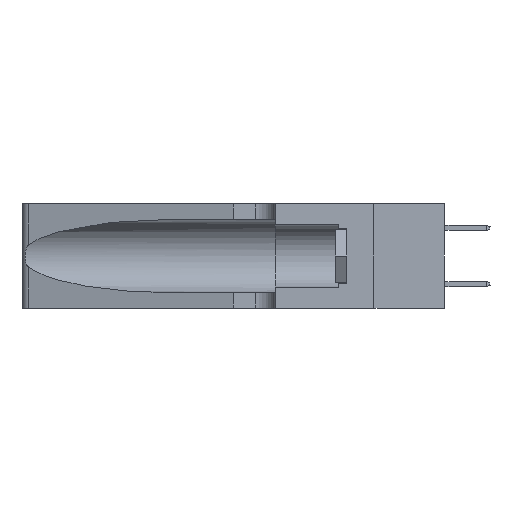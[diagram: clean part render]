
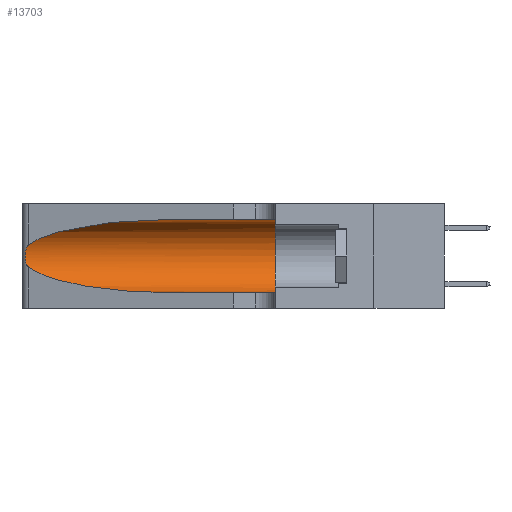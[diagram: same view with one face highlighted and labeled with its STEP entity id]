
A CAD part, left-side view. The second image highlights one B-rep face of the part: STEP entity #13703.
In plain terms, the highlighted cylindrical face has radius 3.308 mm (diameter 6.617 mm), a partial arc.
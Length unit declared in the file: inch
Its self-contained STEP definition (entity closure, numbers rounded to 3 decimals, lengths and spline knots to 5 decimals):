
#345 = ORIENTED_EDGE ( 'NONE', *, *, #11980, .T. ) ;
#488 = VECTOR ( 'NONE', #24105, 39.37008 ) ;
#1249 = CARTESIAN_POINT ( 'NONE',  ( 0.25856, 1.23593, 0.16098 ) ) ;
#1581 = CARTESIAN_POINT ( 'NONE',  ( 0.25639, 1.23184, 0.21858 ) ) ;
#1727 = DIRECTION ( 'NONE',  ( 0., -1., 0. ) ) ;
#2089 = VERTEX_POINT ( 'NONE', #17372 ) ;
#2614 = AXIS2_PLACEMENT_3D ( 'NONE', #23017, #25202, #8219 ) ;
#2866 = CIRCLE ( 'NONE', #2614, 0.13025 ) ;
#4039 = CARTESIAN_POINT ( 'NONE',  ( 0.25789, 1.23486, 0.15765 ) ) ;
#4110 = EDGE_CURVE ( 'NONE', #21217, #9822, #2866, .T. ) ;
#4448 = CARTESIAN_POINT ( 'NONE',  ( 0.2373, 1.15595, 0.08982 ) ) ;
#4817 = CARTESIAN_POINT ( 'NONE',  ( 0.1305, 1.61858, 0.31525 ) ) ;
#6297 = CARTESIAN_POINT ( 'NONE',  ( 0.1305, 0.72297, 0.31525 ) ) ;
#7261 = ORIENTED_EDGE ( 'NONE', *, *, #7979, .F. ) ;
#7979 = EDGE_CURVE ( 'NONE', #8093, #21217, #15474, .T. ) ;
#8093 = VERTEX_POINT ( 'NONE', #6297 ) ;
#8219 = DIRECTION ( 'NONE',  ( 0., 0., 1. ) ) ;
#9145 = CARTESIAN_POINT ( 'NONE',  ( 0.26075, 1.23896, 0.178 ) ) ;
#9822 = VERTEX_POINT ( 'NONE', #28395 ) ;
#11286 = EDGE_CURVE ( 'NONE', #16713, #2089, #21989, .T. ) ;
#11312 = CARTESIAN_POINT ( 'NONE',  ( 0.25555, 1.22994, 0.2215 ) ) ;
#11980 = EDGE_CURVE ( 'NONE', #2089, #9822, #21473, .T. ) ;
#12191 = ORIENTED_EDGE ( 'NONE', *, *, #4110, .F. ) ;
#13606 = DIRECTION ( 'NONE',  ( 0., 0., -1. ) ) ;
#13671 = CARTESIAN_POINT ( 'NONE',  ( 0.25487, 1.22718, 0.22369 ) ) ;
#13703 = ADVANCED_FACE ( 'NONE', ( #27116 ), #22450, .F. ) ;
#13953 = ORIENTED_EDGE ( 'NONE', *, *, #21224, .T. ) ;
#14347 = CARTESIAN_POINT ( 'NONE',  ( 0.25487, 1.22718, 0.14631 ) ) ;
#14461 = CARTESIAN_POINT ( 'NONE',  ( 0.25639, 1.23186, 0.15144 ) ) ;
#15474 = LINE ( 'NONE', #4817, #21306 ) ;
#16266 =( BOUNDED_CURVE ( )  B_SPLINE_CURVE ( 3, ( #28677, #31239, #18958, #13671 ),
 .UNSPECIFIED., .F., .T. ) 
 B_SPLINE_CURVE_WITH_KNOTS ( ( 4, 4 ),
 ( 1.5708, 2.84003 ),
 .UNSPECIFIED. ) 
 CURVE ( )  GEOMETRIC_REPRESENTATION_ITEM ( )  RATIONAL_B_SPLINE_CURVE ( ( 1., 0.87, 0.87, 1. ) ) 
 REPRESENTATION_ITEM ( '' )  );
#16453 = CARTESIAN_POINT ( 'NONE',  ( 0.25487, 1.22718, 0.14631 ) ) ;
#16506 = CARTESIAN_POINT ( 'NONE',  ( 0.1305, 0.35, 0.31525 ) ) ;
#16713 = VERTEX_POINT ( 'NONE', #16453 ) ;
#17372 = CARTESIAN_POINT ( 'NONE',  ( 0.1305, 0.72297, 0.05475 ) ) ;
#18273 = ORIENTED_EDGE ( 'NONE', *, *, #24358, .T. ) ;
#18329 = CARTESIAN_POINT ( 'NONE',  ( 0.1305, 1.61858, 0.05475 ) ) ;
#18750 = CARTESIAN_POINT ( 'NONE',  ( 0.25854, 1.2359, 0.20912 ) ) ;
#18866 = CARTESIAN_POINT ( 'NONE',  ( 0.26075, 1.23896, 0.19203 ) ) ;
#18958 = CARTESIAN_POINT ( 'NONE',  ( 0.2373, 1.15595, 0.28018 ) ) ;
#19444 = B_SPLINE_CURVE_WITH_KNOTS ( 'NONE', 3,
 ( #21134, #11312, #1581, #23953, #18750, #21249, #18866, #9145, #26433, #1249, #4039, #14461, #29241, #14347 ),
 .UNSPECIFIED., .F., .F.,
 ( 4, 2, 2, 2, 2, 2, 4 ),
 ( 0., 0.00027, 0.00053, 0.00107, 0.0016, 0.00187, 0.00214 ),
 .UNSPECIFIED. ) ;
#21134 = CARTESIAN_POINT ( 'NONE',  ( 0.25487, 1.22718, 0.22369 ) ) ;
#21217 = VERTEX_POINT ( 'NONE', #16506 ) ;
#21224 = EDGE_CURVE ( 'NONE', #8093, #24990, #16266, .T. ) ;
#21249 = CARTESIAN_POINT ( 'NONE',  ( 0.26018, 1.23835, 0.19895 ) ) ;
#21306 = VECTOR ( 'NONE', #30594, 39.37008 ) ;
#21473 = LINE ( 'NONE', #18329, #488 ) ;
#21702 = CARTESIAN_POINT ( 'NONE',  ( 0.25487, 1.22718, 0.22369 ) ) ;
#21989 =( BOUNDED_CURVE ( )  B_SPLINE_CURVE ( 3, ( #26277, #4448, #26392, #24242 ),
 .UNSPECIFIED., .F., .F. ) 
 B_SPLINE_CURVE_WITH_KNOTS ( ( 4, 4 ),
 ( 3.44316, 4.71239 ),
 .UNSPECIFIED. ) 
 CURVE ( )  GEOMETRIC_REPRESENTATION_ITEM ( )  RATIONAL_B_SPLINE_CURVE ( ( 1., 0.87, 0.87, 1. ) ) 
 REPRESENTATION_ITEM ( '' )  );
#22450 = CYLINDRICAL_SURFACE ( 'NONE', #23527, 0.13025 ) ;
#23017 = CARTESIAN_POINT ( 'NONE',  ( 0.1305, 0.35, 0.185 ) ) ;
#23527 = AXIS2_PLACEMENT_3D ( 'NONE', #28734, #1727, #13606 ) ;
#23953 = CARTESIAN_POINT ( 'NONE',  ( 0.25787, 1.23484, 0.2124 ) ) ;
#24105 = DIRECTION ( 'NONE',  ( 0., -1., 0. ) ) ;
#24242 = CARTESIAN_POINT ( 'NONE',  ( 0.1305, 0.72297, 0.05475 ) ) ;
#24358 = EDGE_CURVE ( 'NONE', #24990, #16713, #19444, .T. ) ;
#24990 = VERTEX_POINT ( 'NONE', #21702 ) ;
#25202 = DIRECTION ( 'NONE',  ( 0., 1., 0. ) ) ;
#25975 = ORIENTED_EDGE ( 'NONE', *, *, #11286, .T. ) ;
#26277 = CARTESIAN_POINT ( 'NONE',  ( 0.25487, 1.22718, 0.14631 ) ) ;
#26392 = CARTESIAN_POINT ( 'NONE',  ( 0.18966, 0.96281, 0.05475 ) ) ;
#26433 = CARTESIAN_POINT ( 'NONE',  ( 0.26017, 1.23833, 0.17102 ) ) ;
#27116 = FACE_OUTER_BOUND ( 'NONE', #28129, .T. ) ;
#28129 = EDGE_LOOP ( 'NONE', ( #13953, #18273, #25975, #345, #12191, #7261 ) ) ;
#28395 = CARTESIAN_POINT ( 'NONE',  ( 0.1305, 0.35, 0.05475 ) ) ;
#28677 = CARTESIAN_POINT ( 'NONE',  ( 0.1305, 0.72297, 0.31525 ) ) ;
#28734 = CARTESIAN_POINT ( 'NONE',  ( 0.1305, 1.61858, 0.185 ) ) ;
#29241 = CARTESIAN_POINT ( 'NONE',  ( 0.25555, 1.22993, 0.14849 ) ) ;
#30594 = DIRECTION ( 'NONE',  ( 0., -1., 0. ) ) ;
#31239 = CARTESIAN_POINT ( 'NONE',  ( 0.18966, 0.96281, 0.31525 ) ) ;
